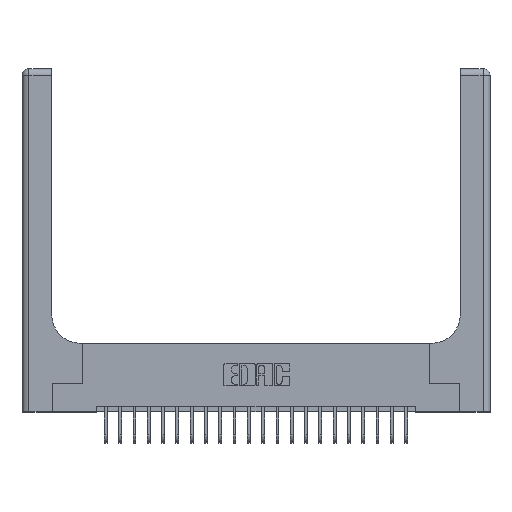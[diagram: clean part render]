
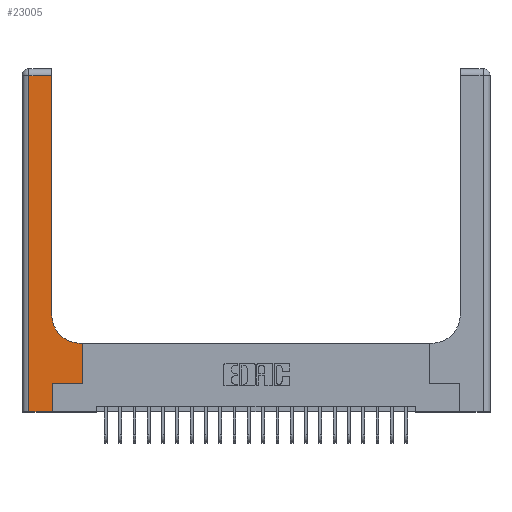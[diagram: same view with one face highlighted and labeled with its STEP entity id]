
A CAD part, top view. The second image highlights one B-rep face of the part: STEP entity #23005.
In plain terms, the highlighted planar face has unit normal (0, 0, 1).
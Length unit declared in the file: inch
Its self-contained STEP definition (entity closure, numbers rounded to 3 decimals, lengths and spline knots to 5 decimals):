
#245 = ORIENTED_EDGE ( 'NONE', *, *, #10038, .T. ) ;
#529 = DIRECTION ( 'NONE',  ( 1., 0., 0. ) ) ;
#677 = CARTESIAN_POINT ( 'NONE',  ( 0.51, 0.6, 0.37 ) ) ;
#680 = CARTESIAN_POINT ( 'NONE',  ( 0.528, 0.6, 0.37 ) ) ;
#872 = VERTEX_POINT ( 'NONE', #11100 ) ;
#901 = VERTEX_POINT ( 'NONE', #680 ) ;
#1498 = CARTESIAN_POINT ( 'NONE',  ( 0., 2.94, 0.37 ) ) ;
#1876 = LINE ( 'NONE', #7589, #5816 ) ;
#1877 = VERTEX_POINT ( 'NONE', #24096 ) ;
#2522 = CARTESIAN_POINT ( 'NONE',  ( 0.528, 0.25, 0.37 ) ) ;
#3346 = AXIS2_PLACEMENT_3D ( 'NONE', #23046, #19417, #529 ) ;
#3943 = EDGE_CURVE ( 'NONE', #16371, #901, #23339, .T. ) ;
#4082 = EDGE_CURVE ( 'NONE', #17964, #24343, #6520, .T. ) ;
#4902 = CARTESIAN_POINT ( 'NONE',  ( 0.06, 0., 0.37 ) ) ;
#5596 = CARTESIAN_POINT ( 'NONE',  ( 0.26, 0.85, 0.37 ) ) ;
#5663 = DIRECTION ( 'NONE',  ( 1., 0., 0. ) ) ;
#5816 = VECTOR ( 'NONE', #13173, 39.37008 ) ;
#5867 = VECTOR ( 'NONE', #15280, 39.37008 ) ;
#6126 = VECTOR ( 'NONE', #6767, 39.37008 ) ;
#6520 = CIRCLE ( 'NONE', #3346, 0.25 ) ;
#6767 = DIRECTION ( 'NONE',  ( 0., 1., 0. ) ) ;
#7589 = CARTESIAN_POINT ( 'NONE',  ( 0.265, 0., 0.37 ) ) ;
#8961 = CARTESIAN_POINT ( 'NONE',  ( 0.265, 0.25, 0.37 ) ) ;
#9072 = DIRECTION ( 'NONE',  ( -1., 0., 0. ) ) ;
#9309 = VECTOR ( 'NONE', #9742, 39.37008 ) ;
#9400 = EDGE_LOOP ( 'NONE', ( #10005, #14423, #10174, #245, #15947, #10659, #22013, #15100, #18578 ) ) ;
#9479 = EDGE_CURVE ( 'NONE', #22123, #19394, #24392, .T. ) ;
#9590 = AXIS2_PLACEMENT_3D ( 'NONE', #14640, #16604, #14404 ) ;
#9742 = DIRECTION ( 'NONE',  ( 0., 1., 0. ) ) ;
#10005 = ORIENTED_EDGE ( 'NONE', *, *, #10491, .T. ) ;
#10038 = EDGE_CURVE ( 'NONE', #10222, #1877, #13584, .T. ) ;
#10174 = ORIENTED_EDGE ( 'NONE', *, *, #11017, .T. ) ;
#10222 = VERTEX_POINT ( 'NONE', #4902 ) ;
#10491 = EDGE_CURVE ( 'NONE', #24343, #22123, #17245, .T. ) ;
#10659 = ORIENTED_EDGE ( 'NONE', *, *, #17467, .T. ) ;
#11017 = EDGE_CURVE ( 'NONE', #19394, #10222, #21427, .T. ) ;
#11100 = CARTESIAN_POINT ( 'NONE',  ( 0.265, 0.25, 0.37 ) ) ;
#11487 = CARTESIAN_POINT ( 'NONE',  ( 0., 0., 0.37 ) ) ;
#12310 = CARTESIAN_POINT ( 'NONE',  ( 0.06, 2.94, 0.37 ) ) ;
#12859 = VECTOR ( 'NONE', #22596, 39.37008 ) ;
#13173 = DIRECTION ( 'NONE',  ( 0., 1., 0. ) ) ;
#13203 = CARTESIAN_POINT ( 'NONE',  ( 0.26, 0.6, 0.37 ) ) ;
#13555 = FACE_OUTER_BOUND ( 'NONE', #9400, .T. ) ;
#13584 = LINE ( 'NONE', #11487, #12859 ) ;
#14022 = VECTOR ( 'NONE', #18960, 39.37008 ) ;
#14404 = DIRECTION ( 'NONE',  ( -1., 0., 0. ) ) ;
#14423 = ORIENTED_EDGE ( 'NONE', *, *, #9479, .T. ) ;
#14640 = CARTESIAN_POINT ( 'NONE',  ( 0., 3., 0.37 ) ) ;
#14786 = VECTOR ( 'NONE', #9072, 39.37008 ) ;
#15100 = ORIENTED_EDGE ( 'NONE', *, *, #19309, .T. ) ;
#15274 = VECTOR ( 'NONE', #5663, 39.37008 ) ;
#15280 = DIRECTION ( 'NONE',  ( -1., 0., 0. ) ) ;
#15947 = ORIENTED_EDGE ( 'NONE', *, *, #17226, .T. ) ;
#16210 = LINE ( 'NONE', #8961, #15274 ) ;
#16371 = VERTEX_POINT ( 'NONE', #2522 ) ;
#16604 = DIRECTION ( 'NONE',  ( 0., 0., -1. ) ) ;
#17226 = EDGE_CURVE ( 'NONE', #1877, #872, #1876, .T. ) ;
#17245 = LINE ( 'NONE', #24453, #9309 ) ;
#17467 = EDGE_CURVE ( 'NONE', #872, #16371, #16210, .T. ) ;
#17964 = VERTEX_POINT ( 'NONE', #677 ) ;
#17986 = CARTESIAN_POINT ( 'NONE',  ( 0.26, 2.94, 0.37 ) ) ;
#18578 = ORIENTED_EDGE ( 'NONE', *, *, #4082, .T. ) ;
#18960 = DIRECTION ( 'NONE',  ( 0., -1., 0. ) ) ;
#19085 = CARTESIAN_POINT ( 'NONE',  ( 0.06, 3., 0.37 ) ) ;
#19309 = EDGE_CURVE ( 'NONE', #901, #17964, #22565, .T. ) ;
#19394 = VERTEX_POINT ( 'NONE', #12310 ) ;
#19417 = DIRECTION ( 'NONE',  ( 0., 0., -1. ) ) ;
#19722 = CARTESIAN_POINT ( 'NONE',  ( 0.528, 0.25, 0.37 ) ) ;
#21064 = PLANE ( 'NONE',  #9590 ) ;
#21427 = LINE ( 'NONE', #19085, #14022 ) ;
#22013 = ORIENTED_EDGE ( 'NONE', *, *, #3943, .T. ) ;
#22123 = VERTEX_POINT ( 'NONE', #17986 ) ;
#22565 = LINE ( 'NONE', #13203, #5867 ) ;
#22596 = DIRECTION ( 'NONE',  ( 1., 0., 0. ) ) ;
#23005 = ADVANCED_FACE ( 'NONE', ( #13555 ), #21064, .F. ) ;
#23046 = CARTESIAN_POINT ( 'NONE',  ( 0.51, 0.85, 0.37 ) ) ;
#23339 = LINE ( 'NONE', #19722, #6126 ) ;
#24096 = CARTESIAN_POINT ( 'NONE',  ( 0.265, 0., 0.37 ) ) ;
#24343 = VERTEX_POINT ( 'NONE', #5596 ) ;
#24392 = LINE ( 'NONE', #1498, #14786 ) ;
#24453 = CARTESIAN_POINT ( 'NONE',  ( 0.26, 3., 0.37 ) ) ;
